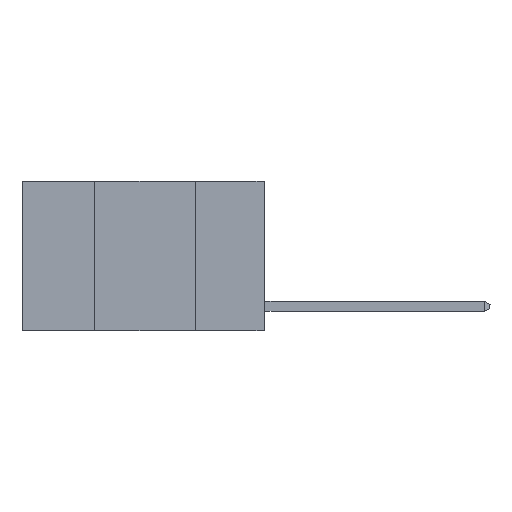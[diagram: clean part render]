
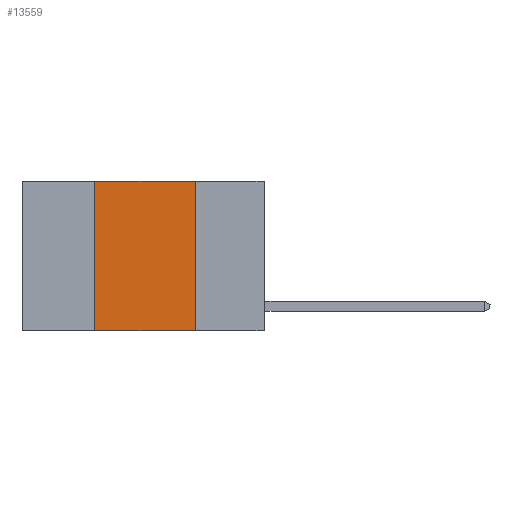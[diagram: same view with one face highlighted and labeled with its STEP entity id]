
A CAD part, left-side view. The second image highlights one B-rep face of the part: STEP entity #13559.
In plain terms, the highlighted planar face has unit normal (-1, 0, 0).
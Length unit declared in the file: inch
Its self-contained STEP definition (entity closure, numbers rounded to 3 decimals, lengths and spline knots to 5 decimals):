
#3 = VERTEX_POINT ( 'NONE', #14569 ) ;
#270 = ORIENTED_EDGE ( 'NONE', *, *, #14940, .F. ) ;
#1483 = PLANE ( 'NONE',  #12614 ) ;
#1886 = EDGE_CURVE ( 'NONE', #3, #6609, #16497, .T. ) ;
#1936 = VERTEX_POINT ( 'NONE', #11272 ) ;
#2678 = CARTESIAN_POINT ( 'NONE',  ( 0., 0.42, 0. ) ) ;
#3875 = CARTESIAN_POINT ( 'NONE',  ( 0., 0.6, 0. ) ) ;
#4328 = VECTOR ( 'NONE', #10429, 39.37008 ) ;
#4454 = DIRECTION ( 'NONE',  ( 0., 0., -1. ) ) ;
#5394 = DIRECTION ( 'NONE',  ( 0., 0., 1. ) ) ;
#6609 = VERTEX_POINT ( 'NONE', #14018 ) ;
#6614 = VERTEX_POINT ( 'NONE', #16676 ) ;
#6832 = CARTESIAN_POINT ( 'NONE',  ( 0., 0.6, 0. ) ) ;
#7244 = EDGE_CURVE ( 'NONE', #6609, #6614, #13466, .T. ) ;
#7384 = CARTESIAN_POINT ( 'NONE',  ( 0., 0.6, -0.37 ) ) ;
#7458 = CARTESIAN_POINT ( 'NONE',  ( 0., 0.17, 0. ) ) ;
#7678 = ORIENTED_EDGE ( 'NONE', *, *, #1886, .F. ) ;
#7762 = EDGE_CURVE ( 'NONE', #3, #1936, #16895, .T. ) ;
#9313 = DIRECTION ( 'NONE',  ( 0., 0., -1. ) ) ;
#9557 = VECTOR ( 'NONE', #4454, 39.37008 ) ;
#10429 = DIRECTION ( 'NONE',  ( 0., -1., 0. ) ) ;
#11272 = CARTESIAN_POINT ( 'NONE',  ( 0., 0.17, -0.37 ) ) ;
#12067 = DIRECTION ( 'NONE',  ( 0., -1., 0. ) ) ;
#12614 = AXIS2_PLACEMENT_3D ( 'NONE', #6832, #16356, #9313 ) ;
#13466 = LINE ( 'NONE', #3875, #13605 ) ;
#13559 = ADVANCED_FACE ( 'NONE', ( #16012 ), #1483, .F. ) ;
#13605 = VECTOR ( 'NONE', #12067, 39.37008 ) ;
#14018 = CARTESIAN_POINT ( 'NONE',  ( 0., 0.42, 0. ) ) ;
#14569 = CARTESIAN_POINT ( 'NONE',  ( 0., 0.42, -0.37 ) ) ;
#14599 = ORIENTED_EDGE ( 'NONE', *, *, #7762, .T. ) ;
#14940 = EDGE_CURVE ( 'NONE', #6614, #1936, #16533, .T. ) ;
#15070 = ORIENTED_EDGE ( 'NONE', *, *, #7244, .F. ) ;
#16012 = FACE_OUTER_BOUND ( 'NONE', #16464, .T. ) ;
#16356 = DIRECTION ( 'NONE',  ( 1., 0., 0. ) ) ;
#16464 = EDGE_LOOP ( 'NONE', ( #270, #15070, #7678, #14599 ) ) ;
#16497 = LINE ( 'NONE', #2678, #17068 ) ;
#16533 = LINE ( 'NONE', #7458, #9557 ) ;
#16676 = CARTESIAN_POINT ( 'NONE',  ( 0., 0.17, 0. ) ) ;
#16895 = LINE ( 'NONE', #7384, #4328 ) ;
#17068 = VECTOR ( 'NONE', #5394, 39.37008 ) ;
